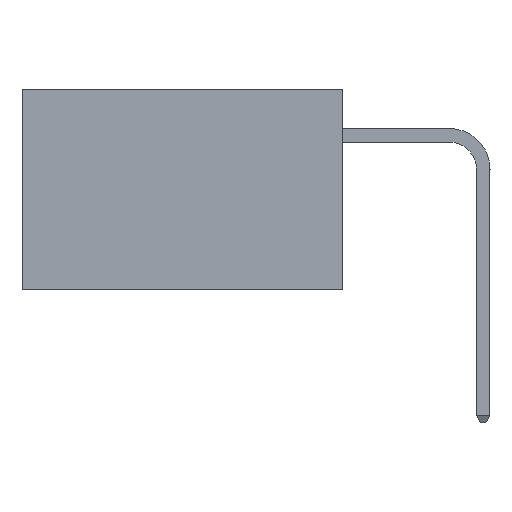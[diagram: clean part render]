
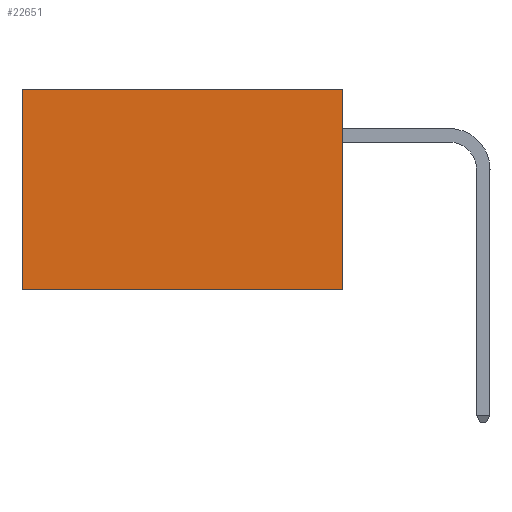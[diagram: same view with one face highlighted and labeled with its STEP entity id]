
A CAD part, left-side view. The second image highlights one B-rep face of the part: STEP entity #22651.
In plain terms, the highlighted planar face has unit normal (-1, 0, 0).
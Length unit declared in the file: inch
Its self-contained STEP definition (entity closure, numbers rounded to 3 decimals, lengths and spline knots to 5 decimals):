
#233 = CARTESIAN_POINT ( 'NONE',  ( 0.277, 0., 0. ) ) ;
#1920 = EDGE_CURVE ( 'NONE', #18563, #10151, #12549, .T. ) ;
#2238 = VERTEX_POINT ( 'NONE', #5430 ) ;
#2845 = VECTOR ( 'NONE', #17356, 39.37008 ) ;
#3431 = CARTESIAN_POINT ( 'NONE',  ( 0.277, 0., -0.37 ) ) ;
#5247 = DIRECTION ( 'NONE',  ( 0., 0., -1. ) ) ;
#5430 = CARTESIAN_POINT ( 'NONE',  ( 0.277, 0.59, -0.37 ) ) ;
#5473 = CARTESIAN_POINT ( 'NONE',  ( 0.277, 0., 0. ) ) ;
#5546 = DIRECTION ( 'NONE',  ( 0., 0., -1. ) ) ;
#5803 = AXIS2_PLACEMENT_3D ( 'NONE', #3431, #16112, #5247 ) ;
#6300 = ORIENTED_EDGE ( 'NONE', *, *, #21403, .T. ) ;
#6438 = LINE ( 'NONE', #7317, #10706 ) ;
#6605 = DIRECTION ( 'NONE',  ( 0., 0., -1. ) ) ;
#7317 = CARTESIAN_POINT ( 'NONE',  ( 0.277, 0.59, -0.37 ) ) ;
#8650 = ORIENTED_EDGE ( 'NONE', *, *, #1920, .T. ) ;
#8692 = CARTESIAN_POINT ( 'NONE',  ( 0.277, 0.59, 0. ) ) ;
#9179 = VERTEX_POINT ( 'NONE', #18561 ) ;
#9465 = ORIENTED_EDGE ( 'NONE', *, *, #11532, .F. ) ;
#10055 = EDGE_CURVE ( 'NONE', #18563, #9179, #10406, .T. ) ;
#10151 = VERTEX_POINT ( 'NONE', #8692 ) ;
#10406 = LINE ( 'NONE', #22765, #19425 ) ;
#10599 = EDGE_LOOP ( 'NONE', ( #6300, #9465, #16095, #8650 ) ) ;
#10706 = VECTOR ( 'NONE', #5546, 39.37008 ) ;
#11532 = EDGE_CURVE ( 'NONE', #9179, #2238, #19285, .T. ) ;
#12345 = DIRECTION ( 'NONE',  ( 0., 1., 0. ) ) ;
#12549 = LINE ( 'NONE', #233, #2845 ) ;
#14329 = PLANE ( 'NONE',  #5803 ) ;
#14533 = VECTOR ( 'NONE', #12345, 39.37008 ) ;
#15995 = FACE_OUTER_BOUND ( 'NONE', #10599, .T. ) ;
#16095 = ORIENTED_EDGE ( 'NONE', *, *, #10055, .F. ) ;
#16112 = DIRECTION ( 'NONE',  ( 1., 0., 0. ) ) ;
#17356 = DIRECTION ( 'NONE',  ( 0., 1., 0. ) ) ;
#18561 = CARTESIAN_POINT ( 'NONE',  ( 0.277, 0., -0.37 ) ) ;
#18563 = VERTEX_POINT ( 'NONE', #5473 ) ;
#19285 = LINE ( 'NONE', #23011, #14533 ) ;
#19425 = VECTOR ( 'NONE', #6605, 39.37008 ) ;
#21403 = EDGE_CURVE ( 'NONE', #10151, #2238, #6438, .T. ) ;
#22651 = ADVANCED_FACE ( 'NONE', ( #15995 ), #14329, .F. ) ;
#22765 = CARTESIAN_POINT ( 'NONE',  ( 0.277, 0., -0.37 ) ) ;
#23011 = CARTESIAN_POINT ( 'NONE',  ( 0.277, 0., -0.37 ) ) ;
